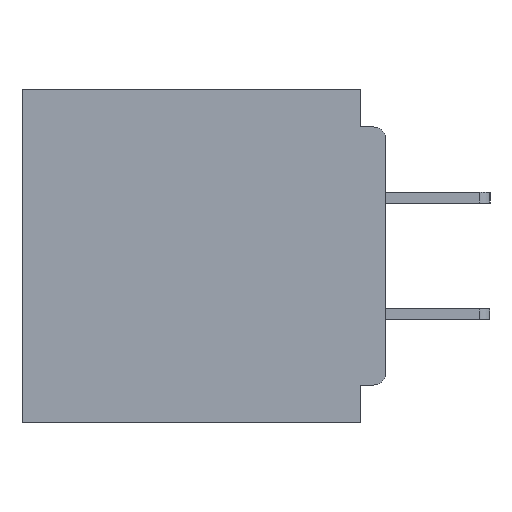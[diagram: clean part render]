
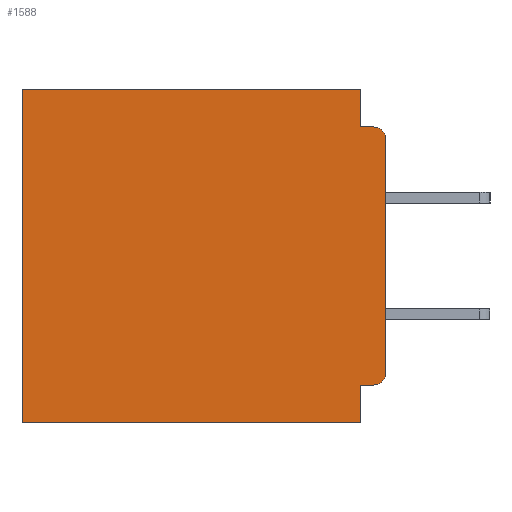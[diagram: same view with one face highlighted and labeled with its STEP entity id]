
A CAD part, left-side view. The second image highlights one B-rep face of the part: STEP entity #1588.
In plain terms, the highlighted planar face has unit normal (-1, 0, 0).
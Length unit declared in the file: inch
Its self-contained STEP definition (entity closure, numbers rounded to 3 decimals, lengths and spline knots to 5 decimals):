
#793 = ORIENTED_EDGE ( 'NONE', *, *, #35319, .F. ) ;
#1422 = FACE_OUTER_BOUND ( 'NONE', #27050, .T. ) ;
#1588 = ADVANCED_FACE ( 'NONE', ( #1422 ), #32431, .F. ) ;
#1703 = AXIS2_PLACEMENT_3D ( 'NONE', #24655, #8251, #27385 ) ;
#2220 = VECTOR ( 'NONE', #11993, 39.37008 ) ;
#2226 = VERTEX_POINT ( 'NONE', #30293 ) ;
#2234 = DIRECTION ( 'NONE',  ( -1., 0., 0. ) ) ;
#2538 = VECTOR ( 'NONE', #3397, 39.37008 ) ;
#3054 = EDGE_CURVE ( 'NONE', #2226, #18509, #20802, .T. ) ;
#3283 = CARTESIAN_POINT ( 'NONE',  ( 0.3, 0.031, -0.4 ) ) ;
#3397 = DIRECTION ( 'NONE',  ( 0., 0., -1. ) ) ;
#3465 = CARTESIAN_POINT ( 'NONE',  ( 0.3, 0., -0.045 ) ) ;
#3661 = CARTESIAN_POINT ( 'NONE',  ( 0.3, 0., -0.4 ) ) ;
#3924 = LINE ( 'NONE', #12859, #17890 ) ;
#4390 = CARTESIAN_POINT ( 'NONE',  ( 0.3, 0.015, -0.045 ) ) ;
#4481 = DIRECTION ( 'NONE',  ( 0., 0., -1. ) ) ;
#5418 = CARTESIAN_POINT ( 'NONE',  ( 0.3, 0., -0.4 ) ) ;
#5774 = CARTESIAN_POINT ( 'NONE',  ( 0.3, 0.031, 0. ) ) ;
#5783 = VECTOR ( 'NONE', #22032, 39.37008 ) ;
#5859 = EDGE_CURVE ( 'NONE', #6413, #33861, #16161, .T. ) ;
#6157 = VECTOR ( 'NONE', #8680, 39.37008 ) ;
#6413 = VERTEX_POINT ( 'NONE', #18198 ) ;
#8251 = DIRECTION ( 'NONE',  ( -1., 0., 0. ) ) ;
#8304 = EDGE_CURVE ( 'NONE', #11857, #2226, #30405, .T. ) ;
#8680 = DIRECTION ( 'NONE',  ( 0., -1., 0. ) ) ;
#9550 = ORIENTED_EDGE ( 'NONE', *, *, #16837, .F. ) ;
#10014 = LINE ( 'NONE', #19976, #2538 ) ;
#10127 = EDGE_CURVE ( 'NONE', #6413, #28410, #15893, .T. ) ;
#11857 = VERTEX_POINT ( 'NONE', #31771 ) ;
#11993 = DIRECTION ( 'NONE',  ( 0., 1., 0. ) ) ;
#12072 = EDGE_CURVE ( 'NONE', #21726, #18509, #29112, .T. ) ;
#12586 = VERTEX_POINT ( 'NONE', #25401 ) ;
#12785 = ORIENTED_EDGE ( 'NONE', *, *, #3054, .F. ) ;
#12859 = CARTESIAN_POINT ( 'NONE',  ( 0.3, 0.437, -0.4 ) ) ;
#12953 = ORIENTED_EDGE ( 'NONE', *, *, #34445, .T. ) ;
#13814 = ORIENTED_EDGE ( 'NONE', *, *, #5859, .F. ) ;
#15127 = DIRECTION ( 'NONE',  ( 0., 1., 0. ) ) ;
#15893 = CIRCLE ( 'NONE', #30478, 0.015 ) ;
#15979 = CARTESIAN_POINT ( 'NONE',  ( 0.3, 0., -0.355 ) ) ;
#16161 = LINE ( 'NONE', #15979, #29686 ) ;
#16295 = EDGE_CURVE ( 'NONE', #33861, #20611, #10014, .T. ) ;
#16837 = EDGE_CURVE ( 'NONE', #21726, #28410, #20445, .T. ) ;
#16868 = CARTESIAN_POINT ( 'NONE',  ( 0.3, 0., -0.34 ) ) ;
#17076 = LINE ( 'NONE', #3661, #2220 ) ;
#17504 = ORIENTED_EDGE ( 'NONE', *, *, #8304, .F. ) ;
#17890 = VECTOR ( 'NONE', #4481, 39.37008 ) ;
#18198 = CARTESIAN_POINT ( 'NONE',  ( 0.3, 0.015, -0.355 ) ) ;
#18509 = VERTEX_POINT ( 'NONE', #4390 ) ;
#18686 = DIRECTION ( 'NONE',  ( 0., 1., 0. ) ) ;
#18880 = CARTESIAN_POINT ( 'NONE',  ( 0.3, 0.015, -0.34 ) ) ;
#19364 = CARTESIAN_POINT ( 'NONE',  ( 0.3, 0., -0.4 ) ) ;
#19976 = CARTESIAN_POINT ( 'NONE',  ( 0.3, 0.031, -0.4 ) ) ;
#20445 = LINE ( 'NONE', #19364, #5783 ) ;
#20611 = VERTEX_POINT ( 'NONE', #3283 ) ;
#20802 = LINE ( 'NONE', #3465, #6157 ) ;
#20907 = CARTESIAN_POINT ( 'NONE',  ( 0.3, 0., -0.06 ) ) ;
#21539 = DIRECTION ( 'NONE',  ( 0., 0., -1. ) ) ;
#21726 = VERTEX_POINT ( 'NONE', #20907 ) ;
#21906 = ORIENTED_EDGE ( 'NONE', *, *, #16295, .F. ) ;
#22032 = DIRECTION ( 'NONE',  ( 0., 0., -1. ) ) ;
#22038 = ORIENTED_EDGE ( 'NONE', *, *, #12072, .T. ) ;
#22247 = DIRECTION ( 'NONE',  ( 0., 0., -1. ) ) ;
#23172 = VECTOR ( 'NONE', #22247, 39.37008 ) ;
#24400 = EDGE_CURVE ( 'NONE', #12586, #27038, #3924, .T. ) ;
#24655 = CARTESIAN_POINT ( 'NONE',  ( 0.3, 0.015, -0.06 ) ) ;
#25038 = VECTOR ( 'NONE', #15127, 39.37008 ) ;
#25059 = AXIS2_PLACEMENT_3D ( 'NONE', #5418, #32481, #31074 ) ;
#25401 = CARTESIAN_POINT ( 'NONE',  ( 0.3, 0.437, 0. ) ) ;
#25803 = ORIENTED_EDGE ( 'NONE', *, *, #24400, .T. ) ;
#25888 = LINE ( 'NONE', #28504, #25038 ) ;
#25916 = CARTESIAN_POINT ( 'NONE',  ( 0.3, 0.031, -0.355 ) ) ;
#26830 = CARTESIAN_POINT ( 'NONE',  ( 0.3, 0.437, -0.4 ) ) ;
#27038 = VERTEX_POINT ( 'NONE', #26830 ) ;
#27050 = EDGE_LOOP ( 'NONE', ( #9550, #22038, #12785, #17504, #12953, #25803, #793, #21906, #13814, #34444 ) ) ;
#27385 = DIRECTION ( 'NONE',  ( 0., 0., -1. ) ) ;
#28410 = VERTEX_POINT ( 'NONE', #16868 ) ;
#28504 = CARTESIAN_POINT ( 'NONE',  ( 0.3, 0., 0. ) ) ;
#29112 = CIRCLE ( 'NONE', #1703, 0.015 ) ;
#29686 = VECTOR ( 'NONE', #18686, 39.37008 ) ;
#30293 = CARTESIAN_POINT ( 'NONE',  ( 0.3, 0.031, -0.045 ) ) ;
#30405 = LINE ( 'NONE', #5774, #23172 ) ;
#30478 = AXIS2_PLACEMENT_3D ( 'NONE', #18880, #2234, #21539 ) ;
#31074 = DIRECTION ( 'NONE',  ( 0., 0., -1. ) ) ;
#31771 = CARTESIAN_POINT ( 'NONE',  ( 0.3, 0.031, 0. ) ) ;
#32431 = PLANE ( 'NONE',  #25059 ) ;
#32481 = DIRECTION ( 'NONE',  ( 1., 0., 0. ) ) ;
#33861 = VERTEX_POINT ( 'NONE', #25916 ) ;
#34444 = ORIENTED_EDGE ( 'NONE', *, *, #10127, .T. ) ;
#34445 = EDGE_CURVE ( 'NONE', #11857, #12586, #25888, .T. ) ;
#35319 = EDGE_CURVE ( 'NONE', #20611, #27038, #17076, .T. ) ;
